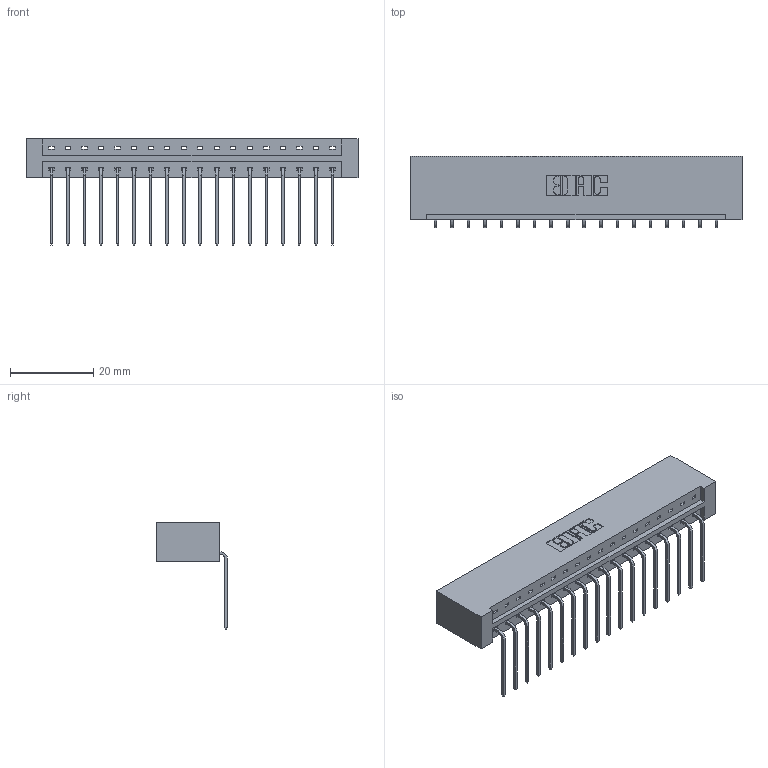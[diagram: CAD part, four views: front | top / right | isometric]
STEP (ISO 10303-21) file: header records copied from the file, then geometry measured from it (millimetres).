
FILE_DESCRIPTION (( 'STEP AP203' ), '1' );
FILE_NAME ('833-018-559-101.STEP', '2020-05-31T23:23:06', ( '' ), ( '' ), 'SwSTEP 2.0', 'SolidWorks 2020', '' );
FILE_SCHEMA (( 'CONFIG_CONTROL_DESIGN' ));
Length unit declared in the file: inch
Products named in the file (3): 345-292-001_558 559 Tail - 1; 833 Part_Lugless; 833-018-559-101
Assembly tree (19 placements, depth 2):
  833-018-559-101
    833 Part_Lugless
    345-292-001_558 559 Tail - 1  x18
Bounding box: 79.58 x 17.09 x 25.53 mm (x, y, z)
Volume: 8474.1 mm3; surface area: 9336 mm2
Topology: 19 solids, 19 shells, 1186 faces, 3563 edges, 2350 vertices
Faces by surface type: plane 858, cylinder 328
Entity records: 13915 total; most frequent: CARTESIAN_POINT 2412, ORIENTED_EDGE 2366, DIRECTION 2075, EDGE_CURVE 1183, VECTOR 1063, LINE 1063, VERTEX_POINT 786, AXIS2_PLACEMENT_3D 506
